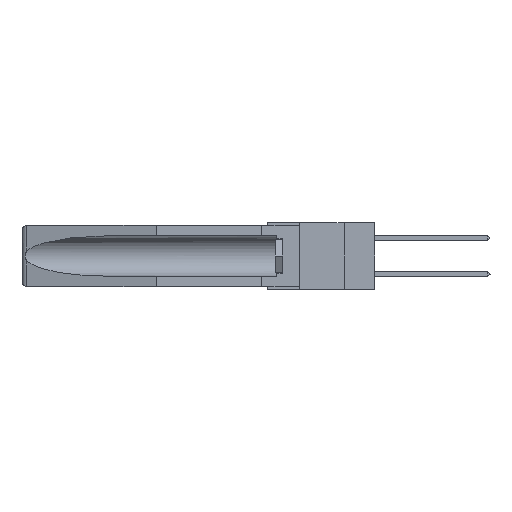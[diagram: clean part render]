
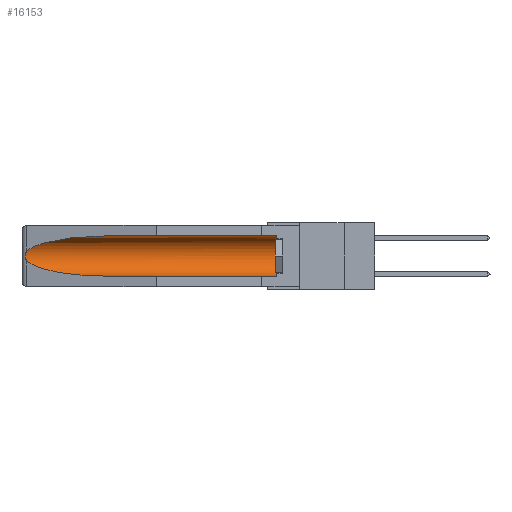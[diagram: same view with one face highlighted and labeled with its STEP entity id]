
A CAD part, left-side view. The second image highlights one B-rep face of the part: STEP entity #16153.
In plain terms, the highlighted cylindrical face has radius 2.857 mm (diameter 5.715 mm), a partial arc.
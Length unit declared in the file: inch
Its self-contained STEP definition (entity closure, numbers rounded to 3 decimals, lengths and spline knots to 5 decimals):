
#1216 = CARTESIAN_POINT ( 'NONE',  ( 0.26597, 1.52961, -0.15275 ) ) ;
#1396 = AXIS2_PLACEMENT_3D ( 'NONE', #6065, #13806, #8003 ) ;
#1875 = CARTESIAN_POINT ( 'NONE',  ( 0.155, 1.07973, -0.284 ) ) ;
#2074 = CARTESIAN_POINT ( 'NONE',  ( 0.26537, 1.52718, -0.14972 ) ) ;
#3075 = CARTESIAN_POINT ( 'NONE',  ( 0.2675, 1.53308, -0.16763 ) ) ;
#3099 = VECTOR ( 'NONE', #7598, 39.37008 ) ;
#3163 = EDGE_CURVE ( 'NONE', #17092, #16220, #24480, .T. ) ;
#3165 = CARTESIAN_POINT ( 'NONE',  ( 0.26537, 1.52718, -0.19328 ) ) ;
#3555 = CARTESIAN_POINT ( 'NONE',  ( 0.26537, 1.52718, -0.19328 ) ) ;
#4150 = ORIENTED_EDGE ( 'NONE', *, *, #9736, .T. ) ;
#4184 = DIRECTION ( 'NONE',  ( 0., 1., 0. ) ) ;
#6065 = CARTESIAN_POINT ( 'NONE',  ( 0.155, -0.30754, -0.1715 ) ) ;
#7153 = CARTESIAN_POINT ( 'NONE',  ( 0.155, 1.07973, -0.059 ) ) ;
#7598 = DIRECTION ( 'NONE',  ( 0., 1., 0. ) ) ;
#7680 = CARTESIAN_POINT ( 'NONE',  ( 0.155, -0.30754, -0.059 ) ) ;
#8003 = DIRECTION ( 'NONE',  ( 0., 0., 1. ) ) ;
#8664 = CARTESIAN_POINT ( 'NONE',  ( 0.26597, 1.5296, -0.19026 ) ) ;
#8944 = CARTESIAN_POINT ( 'NONE',  ( 0.21114, 1.30732, -0.059 ) ) ;
#9312 = CARTESIAN_POINT ( 'NONE',  ( 0.25451, 1.48313, -0.24835 ) ) ;
#9575 = VECTOR ( 'NONE', #4184, 39.37008 ) ;
#9736 = EDGE_CURVE ( 'NONE', #10812, #13010, #18910, .T. ) ;
#9778 = ORIENTED_EDGE ( 'NONE', *, *, #18810, .F. ) ;
#10298 = CIRCLE ( 'NONE', #17082, 0.1125 ) ;
#10600 = CARTESIAN_POINT ( 'NONE',  ( 0.26654, 1.53092, -0.15636 ) ) ;
#10772 = EDGE_CURVE ( 'NONE', #20398, #13396, #10298, .T. ) ;
#10812 = VERTEX_POINT ( 'NONE', #20377 ) ;
#11208 = ORIENTED_EDGE ( 'NONE', *, *, #10772, .T. ) ;
#11484 = LINE ( 'NONE', #7680, #3099 ) ;
#12749 = CARTESIAN_POINT ( 'NONE',  ( 0.155, 1.07973, -0.059 ) ) ;
#13010 = VERTEX_POINT ( 'NONE', #14791 ) ;
#13252 = B_SPLINE_CURVE_WITH_KNOTS ( 'NONE', 3,
 ( #16561, #1216, #10600, #20434, #3075, #24133, #24047, #18232, #8664, #3165 ),
 .UNSPECIFIED., .F., .F.,
 ( 4, 2, 2, 2, 4 ),
 ( 0., 0.00029, 0.00058, 0.00087, 0.00117 ),
 .UNSPECIFIED. ) ;
#13396 = VERTEX_POINT ( 'NONE', #15189 ) ;
#13507 = CARTESIAN_POINT ( 'NONE',  ( 0.155, -0.30754, -0.284 ) ) ;
#13806 = DIRECTION ( 'NONE',  ( 0., 1., 0. ) ) ;
#14736 = DIRECTION ( 'NONE',  ( 0., 0., 1. ) ) ;
#14779 = CYLINDRICAL_SURFACE ( 'NONE', #1396, 0.1125 ) ;
#14791 = CARTESIAN_POINT ( 'NONE',  ( 0.155, 1.07973, -0.284 ) ) ;
#15189 = CARTESIAN_POINT ( 'NONE',  ( 0.155, 0.126, -0.059 ) ) ;
#15224 = ORIENTED_EDGE ( 'NONE', *, *, #3163, .T. ) ;
#15397 = FACE_OUTER_BOUND ( 'NONE', #22473, .T. ) ;
#15902 = ORIENTED_EDGE ( 'NONE', *, *, #24122, .T. ) ;
#16100 = EDGE_CURVE ( 'NONE', #13396, #17092, #11484, .T. ) ;
#16153 = ADVANCED_FACE ( 'NONE', ( #15397 ), #14779, .F. ) ;
#16220 = VERTEX_POINT ( 'NONE', #2074 ) ;
#16561 = CARTESIAN_POINT ( 'NONE',  ( 0.26537, 1.52718, -0.14972 ) ) ;
#16600 = CARTESIAN_POINT ( 'NONE',  ( 0.25451, 1.48313, -0.09465 ) ) ;
#16674 = CARTESIAN_POINT ( 'NONE',  ( 0.155, 0.126, -0.1715 ) ) ;
#16760 = CARTESIAN_POINT ( 'NONE',  ( 0.26537, 1.52718, -0.14972 ) ) ;
#17082 = AXIS2_PLACEMENT_3D ( 'NONE', #16674, #20627, #14736 ) ;
#17092 = VERTEX_POINT ( 'NONE', #7153 ) ;
#18232 = CARTESIAN_POINT ( 'NONE',  ( 0.26655, 1.53094, -0.18657 ) ) ;
#18810 = EDGE_CURVE ( 'NONE', #20398, #13010, #19187, .T. ) ;
#18910 =( BOUNDED_CURVE ( )  B_SPLINE_CURVE ( 3, ( #3555, #9312, #22762, #1875 ),
 .UNSPECIFIED., .F., .F. ) 
 B_SPLINE_CURVE_WITH_KNOTS ( ( 4, 4 ),
 ( 0.1948, 1.5708 ),
 .UNSPECIFIED. ) 
 CURVE ( )  GEOMETRIC_REPRESENTATION_ITEM ( )  RATIONAL_B_SPLINE_CURVE ( ( 1., 0.848, 0.848, 1. ) ) 
 REPRESENTATION_ITEM ( '' )  );
#19187 = LINE ( 'NONE', #13507, #9575 ) ;
#20377 = CARTESIAN_POINT ( 'NONE',  ( 0.26537, 1.52718, -0.19328 ) ) ;
#20398 = VERTEX_POINT ( 'NONE', #21840 ) ;
#20434 = CARTESIAN_POINT ( 'NONE',  ( 0.2673, 1.5327, -0.16383 ) ) ;
#20627 = DIRECTION ( 'NONE',  ( 0., -1., 0. ) ) ;
#21840 = CARTESIAN_POINT ( 'NONE',  ( 0.155, 0.126, -0.284 ) ) ;
#21893 = ORIENTED_EDGE ( 'NONE', *, *, #16100, .T. ) ;
#22473 = EDGE_LOOP ( 'NONE', ( #15224, #15902, #4150, #9778, #11208, #21893 ) ) ;
#22762 = CARTESIAN_POINT ( 'NONE',  ( 0.21114, 1.30732, -0.284 ) ) ;
#24047 = CARTESIAN_POINT ( 'NONE',  ( 0.2673, 1.53269, -0.17917 ) ) ;
#24122 = EDGE_CURVE ( 'NONE', #16220, #10812, #13252, .T. ) ;
#24133 = CARTESIAN_POINT ( 'NONE',  ( 0.2675, 1.53308, -0.17534 ) ) ;
#24480 =( BOUNDED_CURVE ( )  B_SPLINE_CURVE ( 3, ( #12749, #8944, #16600, #16760 ),
 .UNSPECIFIED., .F., .T. ) 
 B_SPLINE_CURVE_WITH_KNOTS ( ( 4, 4 ),
 ( 4.71239, 6.08839 ),
 .UNSPECIFIED. ) 
 CURVE ( )  GEOMETRIC_REPRESENTATION_ITEM ( )  RATIONAL_B_SPLINE_CURVE ( ( 1., 0.848, 0.848, 1. ) ) 
 REPRESENTATION_ITEM ( '' )  );
